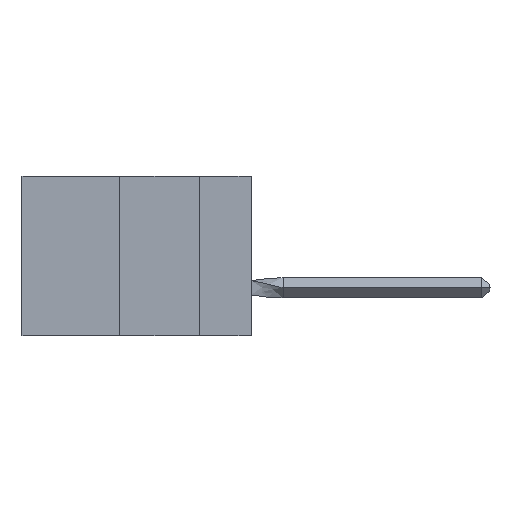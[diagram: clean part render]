
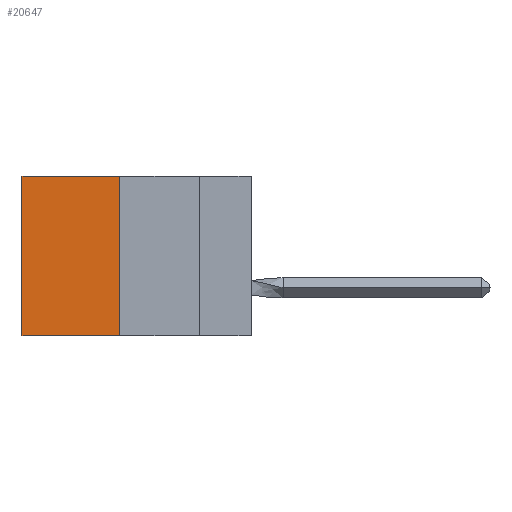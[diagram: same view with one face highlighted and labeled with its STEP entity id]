
A CAD part, left-side view. The second image highlights one B-rep face of the part: STEP entity #20647.
In plain terms, the highlighted planar face has unit normal (-1, 0, 0).
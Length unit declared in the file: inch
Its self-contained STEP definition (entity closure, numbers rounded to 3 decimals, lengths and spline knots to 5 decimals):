
#304 = CARTESIAN_POINT ( 'NONE',  ( 0.305, 0.413, -0.5 ) ) ;
#637 = CARTESIAN_POINT ( 'NONE',  ( 0.305, 0.413, -0.5 ) ) ;
#1656 = LINE ( 'NONE', #27061, #11608 ) ;
#1890 = DIRECTION ( 'NONE',  ( 0., 0., -1. ) ) ;
#2089 = LINE ( 'NONE', #22265, #36386 ) ;
#2307 = AXIS2_PLACEMENT_3D ( 'NONE', #2648, #32778, #32655 ) ;
#2648 = CARTESIAN_POINT ( 'NONE',  ( 0.305, 0.413, -0.5 ) ) ;
#5494 = VERTEX_POINT ( 'NONE', #34973 ) ;
#6993 = CARTESIAN_POINT ( 'NONE',  ( 0.305, 0.72, 0. ) ) ;
#8502 = FACE_OUTER_BOUND ( 'NONE', #13860, .T. ) ;
#11608 = VECTOR ( 'NONE', #33011, 39.37008 ) ;
#11735 = VERTEX_POINT ( 'NONE', #304 ) ;
#13860 = EDGE_LOOP ( 'NONE', ( #38845, #37257, #32677, #25320 ) ) ;
#16680 = EDGE_CURVE ( 'NONE', #5494, #29254, #19172, .T. ) ;
#17788 = CARTESIAN_POINT ( 'NONE',  ( 0.305, 0.72, -0.5 ) ) ;
#18448 = VERTEX_POINT ( 'NONE', #17788 ) ;
#19172 = LINE ( 'NONE', #21975, #19654 ) ;
#19654 = VECTOR ( 'NONE', #21598, 39.37008 ) ;
#20647 = ADVANCED_FACE ( 'NONE', ( #8502 ), #35212, .F. ) ;
#21598 = DIRECTION ( 'NONE',  ( 0., 1., 0. ) ) ;
#21975 = CARTESIAN_POINT ( 'NONE',  ( 0.305, 0.413, 0. ) ) ;
#22265 = CARTESIAN_POINT ( 'NONE',  ( 0.305, 0.72, -0.5 ) ) ;
#23865 = EDGE_CURVE ( 'NONE', #5494, #11735, #28167, .T. ) ;
#24134 = EDGE_CURVE ( 'NONE', #11735, #18448, #1656, .T. ) ;
#25320 = ORIENTED_EDGE ( 'NONE', *, *, #16680, .T. ) ;
#27061 = CARTESIAN_POINT ( 'NONE',  ( 0.305, 0.413, -0.5 ) ) ;
#28167 = LINE ( 'NONE', #637, #36727 ) ;
#29109 = EDGE_CURVE ( 'NONE', #29254, #18448, #2089, .T. ) ;
#29254 = VERTEX_POINT ( 'NONE', #6993 ) ;
#31445 = DIRECTION ( 'NONE',  ( 0., 0., -1. ) ) ;
#32655 = DIRECTION ( 'NONE',  ( 0., 0., -1. ) ) ;
#32677 = ORIENTED_EDGE ( 'NONE', *, *, #23865, .F. ) ;
#32778 = DIRECTION ( 'NONE',  ( 1., 0., 0. ) ) ;
#33011 = DIRECTION ( 'NONE',  ( 0., 1., 0. ) ) ;
#34973 = CARTESIAN_POINT ( 'NONE',  ( 0.305, 0.413, 0. ) ) ;
#35212 = PLANE ( 'NONE',  #2307 ) ;
#36386 = VECTOR ( 'NONE', #1890, 39.37008 ) ;
#36727 = VECTOR ( 'NONE', #31445, 39.37008 ) ;
#37257 = ORIENTED_EDGE ( 'NONE', *, *, #24134, .F. ) ;
#38845 = ORIENTED_EDGE ( 'NONE', *, *, #29109, .T. ) ;
